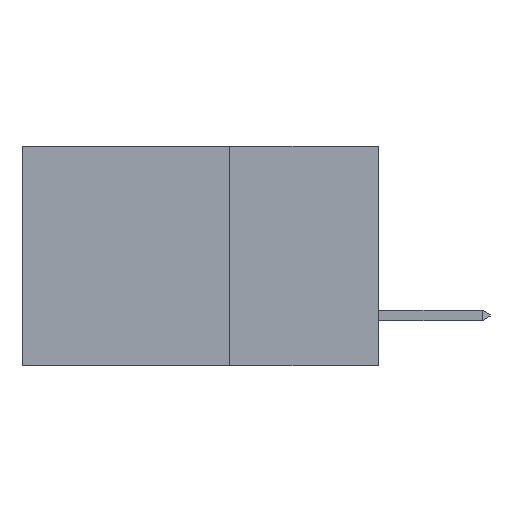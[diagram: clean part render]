
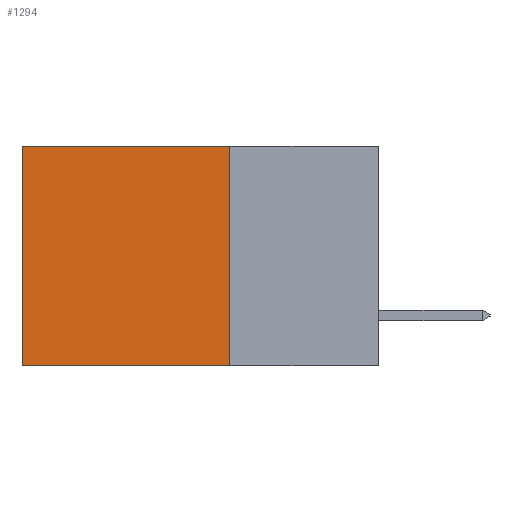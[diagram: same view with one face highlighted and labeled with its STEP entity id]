
A CAD part, left-side view. The second image highlights one B-rep face of the part: STEP entity #1294.
In plain terms, the highlighted planar face has unit normal (-1, 0, 0).
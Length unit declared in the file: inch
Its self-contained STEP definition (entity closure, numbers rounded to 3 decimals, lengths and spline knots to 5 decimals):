
#253 = DIRECTION ( 'NONE',  ( 0., 1., 0. ) ) ;
#1052 = DIRECTION ( 'NONE',  ( 0., 0., -1. ) ) ;
#1294 = ADVANCED_FACE ( 'NONE', ( #10451 ), #8738, .F. ) ;
#1349 = VERTEX_POINT ( 'NONE', #6888 ) ;
#2956 = VECTOR ( 'NONE', #253, 39.37008 ) ;
#3279 = ORIENTED_EDGE ( 'NONE', *, *, #5917, .T. ) ;
#3488 = EDGE_CURVE ( 'NONE', #4394, #11922, #11998, .T. ) ;
#3726 = EDGE_CURVE ( 'NONE', #11922, #1349, #9540, .T. ) ;
#3812 = DIRECTION ( 'NONE',  ( 1., 0., 0. ) ) ;
#4151 = CARTESIAN_POINT ( 'NONE',  ( 0.298, 0.6, 0. ) ) ;
#4244 = CARTESIAN_POINT ( 'NONE',  ( 0.298, 0.25, 0. ) ) ;
#4394 = VERTEX_POINT ( 'NONE', #8339 ) ;
#4410 = VERTEX_POINT ( 'NONE', #6442 ) ;
#4630 = CARTESIAN_POINT ( 'NONE',  ( 0.298, 0.25, 0. ) ) ;
#5130 = EDGE_LOOP ( 'NONE', ( #11793, #11429, #10333, #3279 ) ) ;
#5264 = LINE ( 'NONE', #4151, #12189 ) ;
#5917 = EDGE_CURVE ( 'NONE', #4394, #4410, #10488, .T. ) ;
#6442 = CARTESIAN_POINT ( 'NONE',  ( 0.298, 0.6, 0. ) ) ;
#6826 = EDGE_CURVE ( 'NONE', #4410, #1349, #5264, .T. ) ;
#6888 = CARTESIAN_POINT ( 'NONE',  ( 0.298, 0.6, -0.37 ) ) ;
#7102 = VECTOR ( 'NONE', #11161, 39.37008 ) ;
#7564 = CARTESIAN_POINT ( 'NONE',  ( 0.298, 0.25, 0. ) ) ;
#8044 = DIRECTION ( 'NONE',  ( 0., 0., -1. ) ) ;
#8339 = CARTESIAN_POINT ( 'NONE',  ( 0.298, 0.25, 0. ) ) ;
#8738 = PLANE ( 'NONE',  #9991 ) ;
#9333 = CARTESIAN_POINT ( 'NONE',  ( 0.298, 0.25, -0.37 ) ) ;
#9540 = LINE ( 'NONE', #9757, #7102 ) ;
#9757 = CARTESIAN_POINT ( 'NONE',  ( 0.298, 0.25, -0.37 ) ) ;
#9969 = VECTOR ( 'NONE', #1052, 39.37008 ) ;
#9991 = AXIS2_PLACEMENT_3D ( 'NONE', #7564, #3812, #8044 ) ;
#10333 = ORIENTED_EDGE ( 'NONE', *, *, #3488, .F. ) ;
#10451 = FACE_OUTER_BOUND ( 'NONE', #5130, .T. ) ;
#10488 = LINE ( 'NONE', #4630, #2956 ) ;
#11161 = DIRECTION ( 'NONE',  ( 0., 1., 0. ) ) ;
#11429 = ORIENTED_EDGE ( 'NONE', *, *, #3726, .F. ) ;
#11793 = ORIENTED_EDGE ( 'NONE', *, *, #6826, .T. ) ;
#11922 = VERTEX_POINT ( 'NONE', #9333 ) ;
#11979 = DIRECTION ( 'NONE',  ( 0., 0., -1. ) ) ;
#11998 = LINE ( 'NONE', #4244, #9969 ) ;
#12189 = VECTOR ( 'NONE', #11979, 39.37008 ) ;
